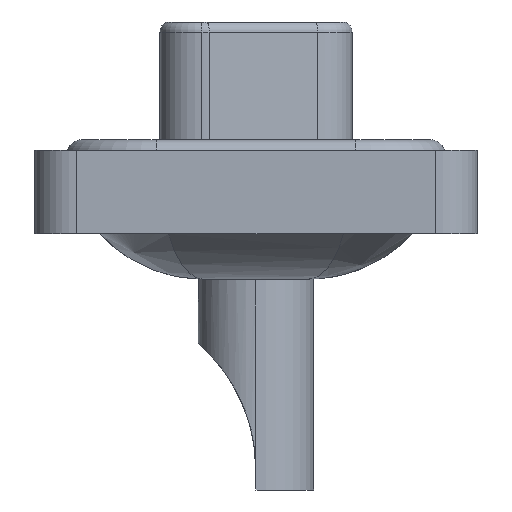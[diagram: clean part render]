
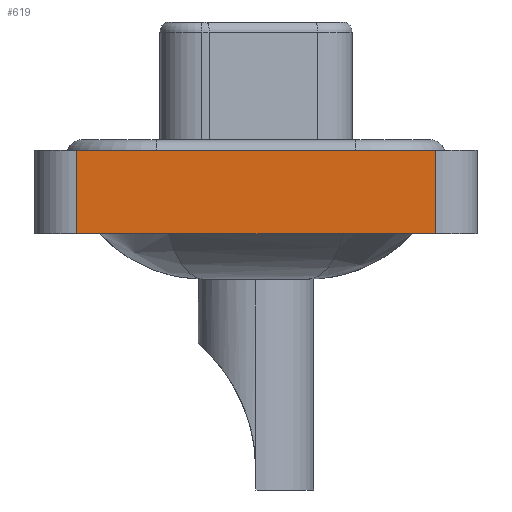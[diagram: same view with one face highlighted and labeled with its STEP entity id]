
A CAD part, left-side view. The second image highlights one B-rep face of the part: STEP entity #619.
In plain terms, the highlighted planar face has unit normal (-1, 0, 0).
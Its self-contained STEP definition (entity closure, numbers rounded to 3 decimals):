
#619 = ADVANCED_FACE ( 'NONE', ( #4033 ), #8667, .T. ) ;
#1317 = DIRECTION ( 'NONE',  ( 0., 0., 1. ) ) ;
#1363 = VERTEX_POINT ( 'NONE', #3136 ) ;
#1467 = LINE ( 'NONE', #10213, #3691 ) ;
#2826 = VECTOR ( 'NONE', #1317, 1000. ) ;
#3136 = CARTESIAN_POINT ( 'NONE',  ( -7.3, -8.55, -3.6 ) ) ;
#3691 = VECTOR ( 'NONE', #15101, 1000. ) ;
#4033 = FACE_OUTER_BOUND ( 'NONE', #8821, .T. ) ;
#4334 = DIRECTION ( 'NONE',  ( 0., 0., 1. ) ) ;
#4860 = VECTOR ( 'NONE', #17494, 1000. ) ;
#5084 = ORIENTED_EDGE ( 'NONE', *, *, #11275, .F. ) ;
#5180 = ORIENTED_EDGE ( 'NONE', *, *, #16261, .F. ) ;
#5275 = VECTOR ( 'NONE', #13165, 1000. ) ;
#5568 = VERTEX_POINT ( 'NONE', #14719 ) ;
#5838 = DIRECTION ( 'NONE',  ( -1., 0., 0. ) ) ;
#8667 = PLANE ( 'NONE',  #10239 ) ;
#8772 = VERTEX_POINT ( 'NONE', #10206 ) ;
#8821 = EDGE_LOOP ( 'NONE', ( #13095, #5084, #5180, #13546 ) ) ;
#9142 = EDGE_CURVE ( 'NONE', #5568, #1363, #14463, .T. ) ;
#10206 = CARTESIAN_POINT ( 'NONE',  ( -7.3, 8.55, 0.4 ) ) ;
#10213 = CARTESIAN_POINT ( 'NONE',  ( -7.3, -8.55, -3.6 ) ) ;
#10239 = AXIS2_PLACEMENT_3D ( 'NONE', #19266, #5838, #4334 ) ;
#10616 = CARTESIAN_POINT ( 'NONE',  ( -7.3, -8.55, 0.4 ) ) ;
#10800 = VERTEX_POINT ( 'NONE', #10616 ) ;
#11275 = EDGE_CURVE ( 'NONE', #8772, #10800, #12587, .T. ) ;
#12587 = LINE ( 'NONE', #15692, #4860 ) ;
#13095 = ORIENTED_EDGE ( 'NONE', *, *, #18177, .T. ) ;
#13165 = DIRECTION ( 'NONE',  ( 0., -1., 0. ) ) ;
#13443 = CARTESIAN_POINT ( 'NONE',  ( -7.3, 8.55, -3.6 ) ) ;
#13546 = ORIENTED_EDGE ( 'NONE', *, *, #9142, .T. ) ;
#14463 = LINE ( 'NONE', #17794, #5275 ) ;
#14719 = CARTESIAN_POINT ( 'NONE',  ( -7.3, 8.55, -3.6 ) ) ;
#15101 = DIRECTION ( 'NONE',  ( 0., 0., 1. ) ) ;
#15692 = CARTESIAN_POINT ( 'NONE',  ( -7.3, -8.55, 0.4 ) ) ;
#16261 = EDGE_CURVE ( 'NONE', #5568, #8772, #19690, .T. ) ;
#17494 = DIRECTION ( 'NONE',  ( 0., -1., 0. ) ) ;
#17794 = CARTESIAN_POINT ( 'NONE',  ( -7.3, -8.55, -3.6 ) ) ;
#18177 = EDGE_CURVE ( 'NONE', #1363, #10800, #1467, .T. ) ;
#19266 = CARTESIAN_POINT ( 'NONE',  ( -7.3, -8.55, -3.6 ) ) ;
#19690 = LINE ( 'NONE', #13443, #2826 ) ;
